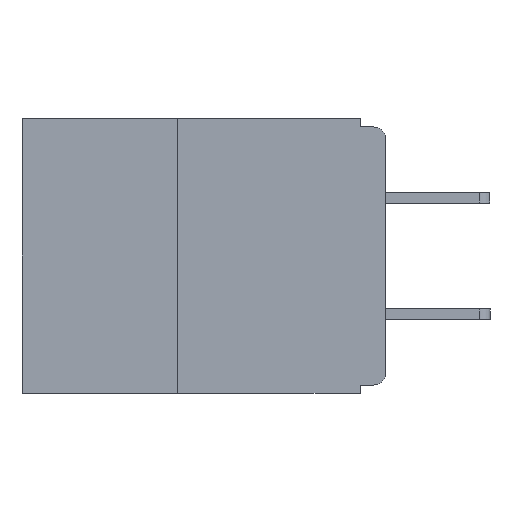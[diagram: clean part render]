
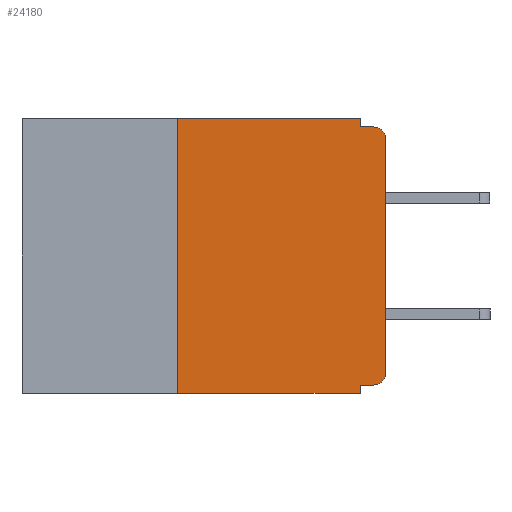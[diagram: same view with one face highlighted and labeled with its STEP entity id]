
A CAD part, left-side view. The second image highlights one B-rep face of the part: STEP entity #24180.
In plain terms, the highlighted planar face has unit normal (-1, 0, 0).
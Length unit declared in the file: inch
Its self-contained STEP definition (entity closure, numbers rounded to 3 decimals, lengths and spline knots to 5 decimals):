
#72 = CARTESIAN_POINT ( 'NONE',  ( 0., 0.25, -0.33 ) ) ;
#645 = VERTEX_POINT ( 'NONE', #5576 ) ;
#653 = CARTESIAN_POINT ( 'NONE',  ( 0., 0., -0.305 ) ) ;
#706 = DIRECTION ( 'NONE',  ( 0., 0., -1. ) ) ;
#710 = CARTESIAN_POINT ( 'NONE',  ( 0., 0.25, -0.33 ) ) ;
#750 = AXIS2_PLACEMENT_3D ( 'NONE', #2641, #17202, #4801 ) ;
#878 = CARTESIAN_POINT ( 'NONE',  ( 0., 0.437, -0.33 ) ) ;
#991 = VECTOR ( 'NONE', #18615, 39.37008 ) ;
#1143 = CARTESIAN_POINT ( 'NONE',  ( 0., 0.031, -0.32 ) ) ;
#1286 = ORIENTED_EDGE ( 'NONE', *, *, #15236, .T. ) ;
#1539 = ORIENTED_EDGE ( 'NONE', *, *, #26519, .T. ) ;
#1952 = VERTEX_POINT ( 'NONE', #27230 ) ;
#2032 = ORIENTED_EDGE ( 'NONE', *, *, #21182, .F. ) ;
#2288 = ORIENTED_EDGE ( 'NONE', *, *, #12513, .F. ) ;
#2641 = CARTESIAN_POINT ( 'NONE',  ( 0., 0.015, -0.025 ) ) ;
#2814 = VECTOR ( 'NONE', #6699, 39.37008 ) ;
#3083 = CIRCLE ( 'NONE', #23523, 0.015 ) ;
#3542 = VERTEX_POINT ( 'NONE', #16556 ) ;
#3853 = VERTEX_POINT ( 'NONE', #12132 ) ;
#3957 = EDGE_LOOP ( 'NONE', ( #1286, #1539, #2032, #2288, #5873, #7159, #16595, #16674, #17506, #19542 ) ) ;
#4012 = CARTESIAN_POINT ( 'NONE',  ( 0., 0.031, 0. ) ) ;
#4282 = CARTESIAN_POINT ( 'NONE',  ( 0., 0.031, -0.01 ) ) ;
#4283 = EDGE_CURVE ( 'NONE', #20160, #645, #8363, .T. ) ;
#4712 = CARTESIAN_POINT ( 'NONE',  ( 0., 0.015, -0.01 ) ) ;
#4801 = DIRECTION ( 'NONE',  ( 0., 0., -1. ) ) ;
#5008 = EDGE_CURVE ( 'NONE', #6942, #3542, #7377, .T. ) ;
#5273 = EDGE_CURVE ( 'NONE', #26416, #20160, #21795, .T. ) ;
#5327 = VECTOR ( 'NONE', #22721, 39.37008 ) ;
#5576 = CARTESIAN_POINT ( 'NONE',  ( 0., 0.031, 0. ) ) ;
#5737 = CARTESIAN_POINT ( 'NONE',  ( 0., 0.015, -0.305 ) ) ;
#5873 = ORIENTED_EDGE ( 'NONE', *, *, #4283, .F. ) ;
#6327 = VERTEX_POINT ( 'NONE', #4282 ) ;
#6699 = DIRECTION ( 'NONE',  ( 0., -1., 0. ) ) ;
#6724 = CARTESIAN_POINT ( 'NONE',  ( 0., 0.437, 0. ) ) ;
#6802 = VERTEX_POINT ( 'NONE', #653 ) ;
#6874 = LINE ( 'NONE', #6967, #11696 ) ;
#6942 = VERTEX_POINT ( 'NONE', #1143 ) ;
#6967 = CARTESIAN_POINT ( 'NONE',  ( 0., 0., -0.32 ) ) ;
#7159 = ORIENTED_EDGE ( 'NONE', *, *, #5273, .F. ) ;
#7377 = LINE ( 'NONE', #16128, #17777 ) ;
#7754 = DIRECTION ( 'NONE',  ( 0., 0., 1. ) ) ;
#7798 = DIRECTION ( 'NONE',  ( 0., 0., -1. ) ) ;
#8067 = CARTESIAN_POINT ( 'NONE',  ( 0., 0., -0.01 ) ) ;
#8082 = EDGE_CURVE ( 'NONE', #26416, #3542, #22570, .T. ) ;
#8363 = LINE ( 'NONE', #6724, #2814 ) ;
#9139 = PLANE ( 'NONE',  #24858 ) ;
#10140 = LINE ( 'NONE', #8067, #5327 ) ;
#10582 = FACE_OUTER_BOUND ( 'NONE', #3957, .T. ) ;
#10733 = VECTOR ( 'NONE', #13431, 39.37008 ) ;
#11696 = VECTOR ( 'NONE', #25782, 39.37008 ) ;
#12132 = CARTESIAN_POINT ( 'NONE',  ( 0., 0.015, -0.32 ) ) ;
#12513 = EDGE_CURVE ( 'NONE', #645, #6327, #17042, .T. ) ;
#13278 = DIRECTION ( 'NONE',  ( 1., 0., 0. ) ) ;
#13431 = DIRECTION ( 'NONE',  ( 0., -1., 0. ) ) ;
#13943 = VECTOR ( 'NONE', #7754, 39.37008 ) ;
#15236 = EDGE_CURVE ( 'NONE', #6802, #1952, #24567, .T. ) ;
#15463 = DIRECTION ( 'NONE',  ( 0., 0., -1. ) ) ;
#16014 = VECTOR ( 'NONE', #27033, 39.37008 ) ;
#16128 = CARTESIAN_POINT ( 'NONE',  ( 0., 0.031, -0.33 ) ) ;
#16556 = CARTESIAN_POINT ( 'NONE',  ( 0., 0.031, -0.33 ) ) ;
#16595 = ORIENTED_EDGE ( 'NONE', *, *, #8082, .T. ) ;
#16674 = ORIENTED_EDGE ( 'NONE', *, *, #5008, .F. ) ;
#17042 = LINE ( 'NONE', #4012, #991 ) ;
#17202 = DIRECTION ( 'NONE',  ( -1., 0., 0. ) ) ;
#17420 = CARTESIAN_POINT ( 'NONE',  ( 0., 0.437, 0. ) ) ;
#17506 = ORIENTED_EDGE ( 'NONE', *, *, #27130, .F. ) ;
#17777 = VECTOR ( 'NONE', #15463, 39.37008 ) ;
#18615 = DIRECTION ( 'NONE',  ( 0., 0., -1. ) ) ;
#18874 = EDGE_CURVE ( 'NONE', #3853, #6802, #3083, .T. ) ;
#19201 = VERTEX_POINT ( 'NONE', #4712 ) ;
#19542 = ORIENTED_EDGE ( 'NONE', *, *, #18874, .T. ) ;
#20160 = VERTEX_POINT ( 'NONE', #24409 ) ;
#20382 = DIRECTION ( 'NONE',  ( -1., 0., 0. ) ) ;
#21182 = EDGE_CURVE ( 'NONE', #6327, #19201, #10140, .T. ) ;
#21795 = LINE ( 'NONE', #710, #16014 ) ;
#22570 = LINE ( 'NONE', #878, #10733 ) ;
#22721 = DIRECTION ( 'NONE',  ( 0., -1., 0. ) ) ;
#23258 = CIRCLE ( 'NONE', #750, 0.015 ) ;
#23523 = AXIS2_PLACEMENT_3D ( 'NONE', #5737, #20382, #7798 ) ;
#24180 = ADVANCED_FACE ( 'NONE', ( #10582 ), #9139, .F. ) ;
#24409 = CARTESIAN_POINT ( 'NONE',  ( 0., 0.25, 0. ) ) ;
#24567 = LINE ( 'NONE', #26557, #13943 ) ;
#24858 = AXIS2_PLACEMENT_3D ( 'NONE', #17420, #13278, #706 ) ;
#25782 = DIRECTION ( 'NONE',  ( 0., 1., 0. ) ) ;
#26416 = VERTEX_POINT ( 'NONE', #72 ) ;
#26519 = EDGE_CURVE ( 'NONE', #1952, #19201, #23258, .T. ) ;
#26557 = CARTESIAN_POINT ( 'NONE',  ( 0., 0., 0. ) ) ;
#27033 = DIRECTION ( 'NONE',  ( 0., 0., 1. ) ) ;
#27130 = EDGE_CURVE ( 'NONE', #3853, #6942, #6874, .T. ) ;
#27230 = CARTESIAN_POINT ( 'NONE',  ( 0., 0., -0.025 ) ) ;
